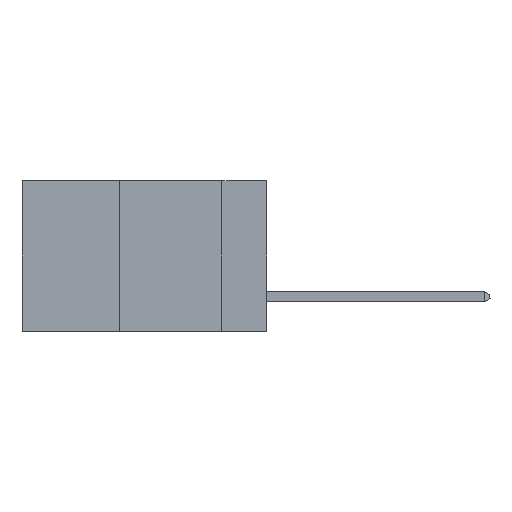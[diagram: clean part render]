
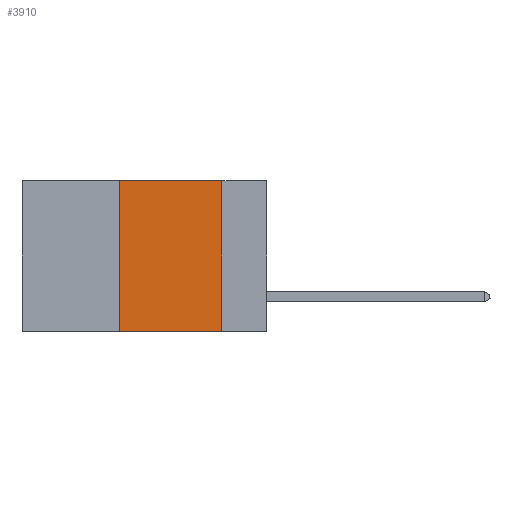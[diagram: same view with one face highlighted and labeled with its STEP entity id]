
A CAD part, left-side view. The second image highlights one B-rep face of the part: STEP entity #3910.
In plain terms, the highlighted planar face has unit normal (-1, 0, 0).
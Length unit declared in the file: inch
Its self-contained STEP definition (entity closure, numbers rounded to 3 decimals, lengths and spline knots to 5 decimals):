
#1762 = LINE ( 'NONE', #31052, #26009 ) ;
#3534 = EDGE_CURVE ( 'NONE', #30962, #26026, #28429, .T. ) ;
#3910 = ADVANCED_FACE ( 'NONE', ( #25173 ), #27176, .F. ) ;
#5857 = EDGE_CURVE ( 'NONE', #26026, #25420, #29678, .T. ) ;
#8777 = LINE ( 'NONE', #9138, #37614 ) ;
#9138 = CARTESIAN_POINT ( 'NONE',  ( 0., 0.36, 0. ) ) ;
#9398 = CARTESIAN_POINT ( 'NONE',  ( 0., 0.6, 0. ) ) ;
#10001 = CARTESIAN_POINT ( 'NONE',  ( 0., 0.11, 0. ) ) ;
#11975 = EDGE_CURVE ( 'NONE', #26874, #30962, #8777, .T. ) ;
#12068 = DIRECTION ( 'NONE',  ( 1., 0., 0. ) ) ;
#12554 = EDGE_LOOP ( 'NONE', ( #13307, #14388, #30796, #23462 ) ) ;
#13307 = ORIENTED_EDGE ( 'NONE', *, *, #5857, .F. ) ;
#14388 = ORIENTED_EDGE ( 'NONE', *, *, #3534, .F. ) ;
#17660 = EDGE_CURVE ( 'NONE', #26874, #25420, #1762, .T. ) ;
#17773 = DIRECTION ( 'NONE',  ( 0., 0., -1. ) ) ;
#18097 = DIRECTION ( 'NONE',  ( 0., 0., -1. ) ) ;
#22992 = AXIS2_PLACEMENT_3D ( 'NONE', #9398, #12068, #18097 ) ;
#23462 = ORIENTED_EDGE ( 'NONE', *, *, #17660, .T. ) ;
#24069 = DIRECTION ( 'NONE',  ( 0., 0., 1. ) ) ;
#24483 = CARTESIAN_POINT ( 'NONE',  ( 0., 0.11, -0.37 ) ) ;
#25173 = FACE_OUTER_BOUND ( 'NONE', #12554, .T. ) ;
#25234 = CARTESIAN_POINT ( 'NONE',  ( 0., 0.36, 0. ) ) ;
#25420 = VERTEX_POINT ( 'NONE', #24483 ) ;
#25734 = CARTESIAN_POINT ( 'NONE',  ( 0., 0.6, 0. ) ) ;
#26009 = VECTOR ( 'NONE', #37087, 39.37008 ) ;
#26026 = VERTEX_POINT ( 'NONE', #10001 ) ;
#26874 = VERTEX_POINT ( 'NONE', #27060 ) ;
#27060 = CARTESIAN_POINT ( 'NONE',  ( 0., 0.36, -0.37 ) ) ;
#27176 = PLANE ( 'NONE',  #22992 ) ;
#27343 = DIRECTION ( 'NONE',  ( 0., -1., 0. ) ) ;
#28429 = LINE ( 'NONE', #25734, #35854 ) ;
#29678 = LINE ( 'NONE', #32580, #32036 ) ;
#30796 = ORIENTED_EDGE ( 'NONE', *, *, #11975, .F. ) ;
#30962 = VERTEX_POINT ( 'NONE', #25234 ) ;
#31052 = CARTESIAN_POINT ( 'NONE',  ( 0., 0.6, -0.37 ) ) ;
#32036 = VECTOR ( 'NONE', #17773, 39.37008 ) ;
#32580 = CARTESIAN_POINT ( 'NONE',  ( 0., 0.11, 0. ) ) ;
#35854 = VECTOR ( 'NONE', #27343, 39.37008 ) ;
#37087 = DIRECTION ( 'NONE',  ( 0., -1., 0. ) ) ;
#37614 = VECTOR ( 'NONE', #24069, 39.37008 ) ;
